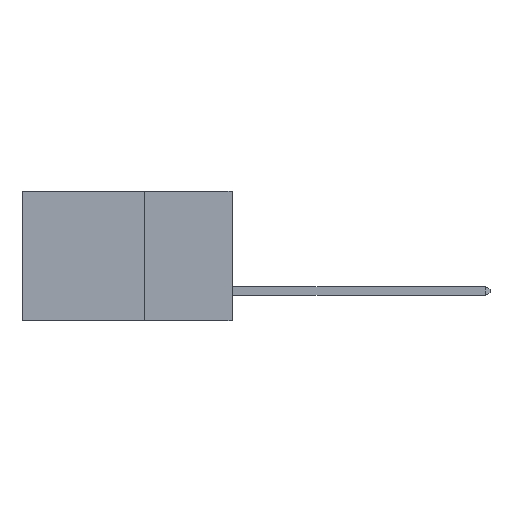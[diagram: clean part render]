
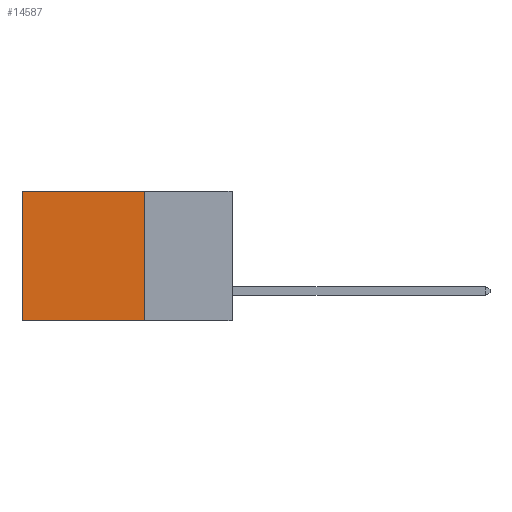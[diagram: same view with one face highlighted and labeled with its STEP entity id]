
A CAD part, left-side view. The second image highlights one B-rep face of the part: STEP entity #14587.
In plain terms, the highlighted planar face has unit normal (-1, 0, 0).
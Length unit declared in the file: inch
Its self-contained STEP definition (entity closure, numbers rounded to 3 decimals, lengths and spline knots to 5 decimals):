
#432 = DIRECTION ( 'NONE',  ( 0., 1., 0. ) ) ;
#993 = LINE ( 'NONE', #15130, #20634 ) ;
#1049 = EDGE_CURVE ( 'NONE', #22469, #35363, #27209, .T. ) ;
#1164 = CARTESIAN_POINT ( 'NONE',  ( 0.2875, 0.25, 0. ) ) ;
#4422 = DIRECTION ( 'NONE',  ( 0., 1., 0. ) ) ;
#4626 = DIRECTION ( 'NONE',  ( 0., 0., -1. ) ) ;
#5168 = AXIS2_PLACEMENT_3D ( 'NONE', #1164, #21101, #4626 ) ;
#5621 = LINE ( 'NONE', #40993, #11252 ) ;
#6911 = ORIENTED_EDGE ( 'NONE', *, *, #26271, .T. ) ;
#7031 = ORIENTED_EDGE ( 'NONE', *, *, #25834, .T. ) ;
#8122 = VECTOR ( 'NONE', #26409, 39.37008 ) ;
#9332 = CARTESIAN_POINT ( 'NONE',  ( 0.2875, 0.25, 0. ) ) ;
#10439 = EDGE_LOOP ( 'NONE', ( #7031, #31075, #32094, #6911 ) ) ;
#10475 = CARTESIAN_POINT ( 'NONE',  ( 0.2875, 0.6, 0. ) ) ;
#11252 = VECTOR ( 'NONE', #4422, 39.37008 ) ;
#12012 = VERTEX_POINT ( 'NONE', #10475 ) ;
#13807 = CARTESIAN_POINT ( 'NONE',  ( 0.2875, 0.25, -0.37 ) ) ;
#13893 = CARTESIAN_POINT ( 'NONE',  ( 0.2875, 0.25, -0.37 ) ) ;
#13909 = VERTEX_POINT ( 'NONE', #24625 ) ;
#14587 = ADVANCED_FACE ( 'NONE', ( #24318 ), #33833, .F. ) ;
#15130 = CARTESIAN_POINT ( 'NONE',  ( 0.2875, 0.6, 0. ) ) ;
#16306 = CARTESIAN_POINT ( 'NONE',  ( 0.2875, 0.25, 0. ) ) ;
#16644 = LINE ( 'NONE', #13807, #30609 ) ;
#19792 = EDGE_CURVE ( 'NONE', #35363, #13909, #16644, .T. ) ;
#20634 = VECTOR ( 'NONE', #21495, 39.37008 ) ;
#21101 = DIRECTION ( 'NONE',  ( 1., 0., 0. ) ) ;
#21495 = DIRECTION ( 'NONE',  ( 0., 0., -1. ) ) ;
#22469 = VERTEX_POINT ( 'NONE', #9332 ) ;
#24318 = FACE_OUTER_BOUND ( 'NONE', #10439, .T. ) ;
#24625 = CARTESIAN_POINT ( 'NONE',  ( 0.2875, 0.6, -0.37 ) ) ;
#25834 = EDGE_CURVE ( 'NONE', #12012, #13909, #993, .T. ) ;
#26271 = EDGE_CURVE ( 'NONE', #22469, #12012, #5621, .T. ) ;
#26409 = DIRECTION ( 'NONE',  ( 0., 0., -1. ) ) ;
#27209 = LINE ( 'NONE', #16306, #8122 ) ;
#30609 = VECTOR ( 'NONE', #432, 39.37008 ) ;
#31075 = ORIENTED_EDGE ( 'NONE', *, *, #19792, .F. ) ;
#32094 = ORIENTED_EDGE ( 'NONE', *, *, #1049, .F. ) ;
#33833 = PLANE ( 'NONE',  #5168 ) ;
#35363 = VERTEX_POINT ( 'NONE', #13893 ) ;
#40993 = CARTESIAN_POINT ( 'NONE',  ( 0.2875, 0.25, 0. ) ) ;
